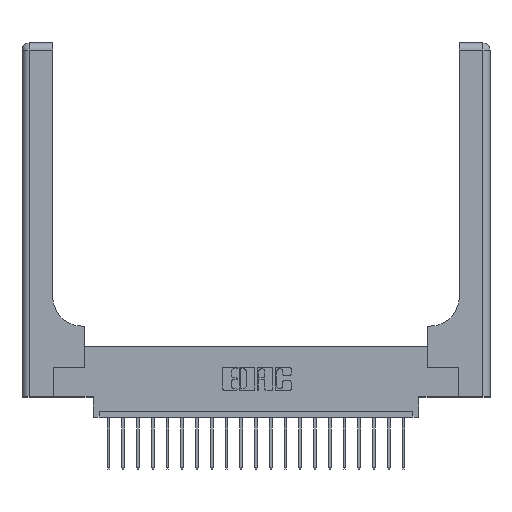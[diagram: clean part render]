
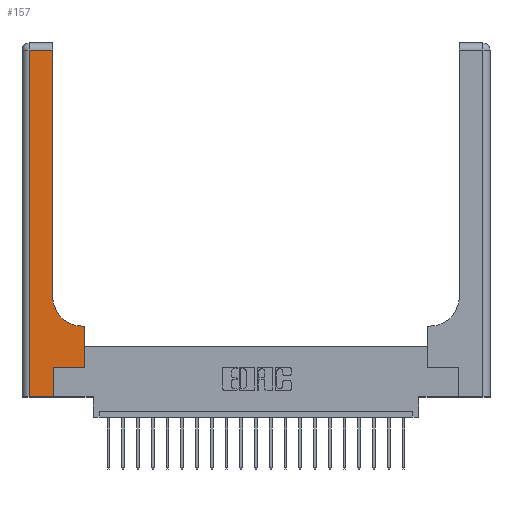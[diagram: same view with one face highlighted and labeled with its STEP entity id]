
A CAD part, top view. The second image highlights one B-rep face of the part: STEP entity #157.
In plain terms, the highlighted planar face has unit normal (0, 0, 1).
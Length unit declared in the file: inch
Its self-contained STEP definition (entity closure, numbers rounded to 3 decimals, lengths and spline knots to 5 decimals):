
#157 = ADVANCED_FACE ( 'NONE', ( #10071 ), #1602, .F. ) ;
#380 = CARTESIAN_POINT ( 'NONE',  ( 0.265, 0.25, 0.37 ) ) ;
#687 = VERTEX_POINT ( 'NONE', #16765 ) ;
#694 = AXIS2_PLACEMENT_3D ( 'NONE', #1530, #11529, #5087 ) ;
#1076 = CARTESIAN_POINT ( 'NONE',  ( 0.26, 0.85, 0.37 ) ) ;
#1530 = CARTESIAN_POINT ( 'NONE',  ( 0., 3., 0.37 ) ) ;
#1602 = PLANE ( 'NONE',  #694 ) ;
#2036 = ORIENTED_EDGE ( 'NONE', *, *, #3383, .T. ) ;
#2056 = LINE ( 'NONE', #12653, #2320 ) ;
#2133 = DIRECTION ( 'NONE',  ( 0., 1., 0. ) ) ;
#2320 = VECTOR ( 'NONE', #11016, 39.37008 ) ;
#2375 = DIRECTION ( 'NONE',  ( 0., -1., 0. ) ) ;
#2451 = CARTESIAN_POINT ( 'NONE',  ( 0.06, 3., 0.37 ) ) ;
#2546 = LINE ( 'NONE', #14974, #11766 ) ;
#3117 = VECTOR ( 'NONE', #2133, 39.37008 ) ;
#3141 = EDGE_CURVE ( 'NONE', #14970, #16855, #17338, .T. ) ;
#3383 = EDGE_CURVE ( 'NONE', #18719, #9108, #18852, .T. ) ;
#3416 = ORIENTED_EDGE ( 'NONE', *, *, #3141, .T. ) ;
#4550 = CARTESIAN_POINT ( 'NONE',  ( 0., 2.94, 0.37 ) ) ;
#4614 = CARTESIAN_POINT ( 'NONE',  ( 0.51, 0.6, 0.37 ) ) ;
#4928 = VERTEX_POINT ( 'NONE', #6202 ) ;
#5087 = DIRECTION ( 'NONE',  ( -1., 0., 0. ) ) ;
#5412 = VERTEX_POINT ( 'NONE', #4614 ) ;
#6202 = CARTESIAN_POINT ( 'NONE',  ( 0.26, 2.94, 0.37 ) ) ;
#6273 = DIRECTION ( 'NONE',  ( 0., 0., -1. ) ) ;
#6416 = VECTOR ( 'NONE', #16375, 39.37008 ) ;
#6572 = CARTESIAN_POINT ( 'NONE',  ( 0.528, 0.25, 0.37 ) ) ;
#7280 = ORIENTED_EDGE ( 'NONE', *, *, #13907, .T. ) ;
#7553 = EDGE_LOOP ( 'NONE', ( #12008, #7280, #2036, #11254, #10622, #3416, #8818, #11651, #15932 ) ) ;
#7652 = DIRECTION ( 'NONE',  ( 0., 1., 0. ) ) ;
#8797 = CARTESIAN_POINT ( 'NONE',  ( 0.06, 2.94, 0.37 ) ) ;
#8818 = ORIENTED_EDGE ( 'NONE', *, *, #16635, .T. ) ;
#9108 = VERTEX_POINT ( 'NONE', #13087 ) ;
#9302 = CIRCLE ( 'NONE', #10407, 0.25 ) ;
#9868 = EDGE_CURVE ( 'NONE', #687, #14970, #13350, .T. ) ;
#10071 = FACE_OUTER_BOUND ( 'NONE', #7553, .T. ) ;
#10407 = AXIS2_PLACEMENT_3D ( 'NONE', #14437, #6273, #12731 ) ;
#10622 = ORIENTED_EDGE ( 'NONE', *, *, #9868, .T. ) ;
#10863 = LINE ( 'NONE', #13329, #15971 ) ;
#11016 = DIRECTION ( 'NONE',  ( 1., 0., 0. ) ) ;
#11254 = ORIENTED_EDGE ( 'NONE', *, *, #15813, .T. ) ;
#11378 = LINE ( 'NONE', #4550, #16242 ) ;
#11471 = DIRECTION ( 'NONE',  ( 0., 1., 0. ) ) ;
#11485 = DIRECTION ( 'NONE',  ( 1., 0., 0. ) ) ;
#11529 = DIRECTION ( 'NONE',  ( 0., 0., -1. ) ) ;
#11651 = ORIENTED_EDGE ( 'NONE', *, *, #16841, .T. ) ;
#11766 = VECTOR ( 'NONE', #11471, 39.37008 ) ;
#12008 = ORIENTED_EDGE ( 'NONE', *, *, #14000, .T. ) ;
#12530 = LINE ( 'NONE', #16163, #6416 ) ;
#12653 = CARTESIAN_POINT ( 'NONE',  ( 0., 0., 0.37 ) ) ;
#12731 = DIRECTION ( 'NONE',  ( 1., 0., 0. ) ) ;
#13011 = VECTOR ( 'NONE', #11485, 39.37008 ) ;
#13087 = CARTESIAN_POINT ( 'NONE',  ( 0.06, 0., 0.37 ) ) ;
#13329 = CARTESIAN_POINT ( 'NONE',  ( 0.26, 3., 0.37 ) ) ;
#13350 = LINE ( 'NONE', #15027, #3117 ) ;
#13437 = VERTEX_POINT ( 'NONE', #1076 ) ;
#13907 = EDGE_CURVE ( 'NONE', #4928, #18719, #11378, .T. ) ;
#14000 = EDGE_CURVE ( 'NONE', #13437, #4928, #10863, .T. ) ;
#14437 = CARTESIAN_POINT ( 'NONE',  ( 0.51, 0.85, 0.37 ) ) ;
#14970 = VERTEX_POINT ( 'NONE', #380 ) ;
#14974 = CARTESIAN_POINT ( 'NONE',  ( 0.528, 0.25, 0.37 ) ) ;
#15027 = CARTESIAN_POINT ( 'NONE',  ( 0.265, 0., 0.37 ) ) ;
#15688 = VERTEX_POINT ( 'NONE', #20736 ) ;
#15813 = EDGE_CURVE ( 'NONE', #9108, #687, #2056, .T. ) ;
#15932 = ORIENTED_EDGE ( 'NONE', *, *, #19171, .T. ) ;
#15971 = VECTOR ( 'NONE', #7652, 39.37008 ) ;
#16163 = CARTESIAN_POINT ( 'NONE',  ( 0.26, 0.6, 0.37 ) ) ;
#16242 = VECTOR ( 'NONE', #19050, 39.37008 ) ;
#16375 = DIRECTION ( 'NONE',  ( -1., 0., 0. ) ) ;
#16635 = EDGE_CURVE ( 'NONE', #16855, #15688, #2546, .T. ) ;
#16765 = CARTESIAN_POINT ( 'NONE',  ( 0.265, 0., 0.37 ) ) ;
#16841 = EDGE_CURVE ( 'NONE', #15688, #5412, #12530, .T. ) ;
#16855 = VERTEX_POINT ( 'NONE', #6572 ) ;
#17338 = LINE ( 'NONE', #19771, #13011 ) ;
#18335 = VECTOR ( 'NONE', #2375, 39.37008 ) ;
#18719 = VERTEX_POINT ( 'NONE', #8797 ) ;
#18852 = LINE ( 'NONE', #2451, #18335 ) ;
#19050 = DIRECTION ( 'NONE',  ( -1., 0., 0. ) ) ;
#19171 = EDGE_CURVE ( 'NONE', #5412, #13437, #9302, .T. ) ;
#19771 = CARTESIAN_POINT ( 'NONE',  ( 0.265, 0.25, 0.37 ) ) ;
#20736 = CARTESIAN_POINT ( 'NONE',  ( 0.528, 0.6, 0.37 ) ) ;
